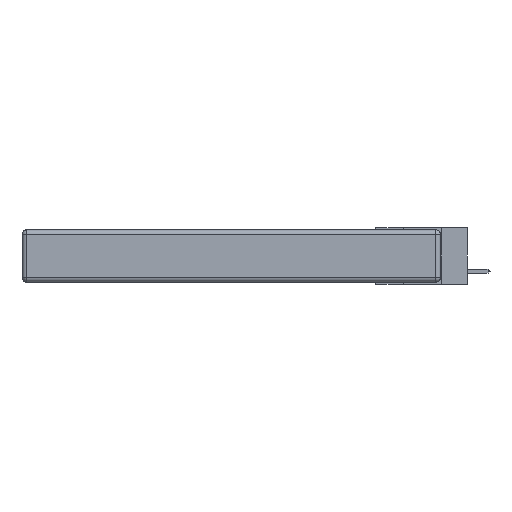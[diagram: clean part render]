
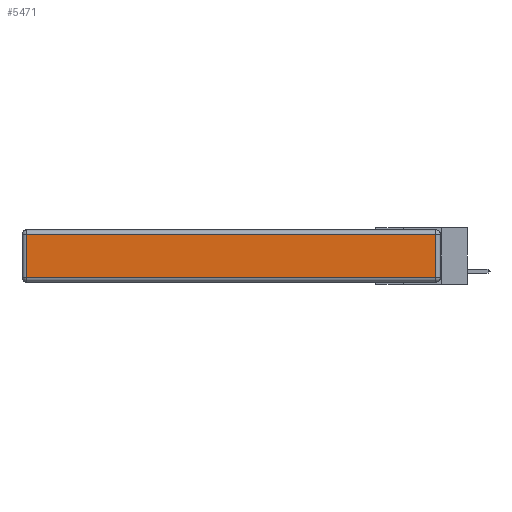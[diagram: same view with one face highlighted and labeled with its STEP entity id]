
A CAD part, left-side view. The second image highlights one B-rep face of the part: STEP entity #5471.
In plain terms, the highlighted planar face has unit normal (-1, 0, 0).
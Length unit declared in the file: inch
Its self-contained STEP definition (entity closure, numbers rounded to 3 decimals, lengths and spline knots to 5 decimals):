
#428 = CARTESIAN_POINT ( 'NONE',  ( 0., 0.03, -0.313 ) ) ;
#911 = EDGE_CURVE ( 'NONE', #13540, #8056, #10536, .T. ) ;
#1095 = VERTEX_POINT ( 'NONE', #428 ) ;
#1838 = ORIENTED_EDGE ( 'NONE', *, *, #20909, .T. ) ;
#2968 = CARTESIAN_POINT ( 'NONE',  ( 0., 2.72, -0.313 ) ) ;
#4421 = DIRECTION ( 'NONE',  ( 0., 1., 0. ) ) ;
#4935 = ORIENTED_EDGE ( 'NONE', *, *, #13201, .T. ) ;
#5303 = DIRECTION ( 'NONE',  ( -1., 0., 0. ) ) ;
#5471 = ADVANCED_FACE ( 'NONE', ( #12807 ), #6971, .T. ) ;
#5778 = AXIS2_PLACEMENT_3D ( 'NONE', #19087, #5303, #8729 ) ;
#5920 = VECTOR ( 'NONE', #4421, 39.37008 ) ;
#6203 = VECTOR ( 'NONE', #10778, 39.37008 ) ;
#6971 = PLANE ( 'NONE',  #5778 ) ;
#7053 = CARTESIAN_POINT ( 'NONE',  ( 0., 0.03, -0.343 ) ) ;
#7237 = CARTESIAN_POINT ( 'NONE',  ( 0., 0., -0.313 ) ) ;
#7710 = VECTOR ( 'NONE', #8641, 39.37008 ) ;
#8056 = VERTEX_POINT ( 'NONE', #19097 ) ;
#8262 = ORIENTED_EDGE ( 'NONE', *, *, #9685, .T. ) ;
#8641 = DIRECTION ( 'NONE',  ( 0., 0., 1. ) ) ;
#8729 = DIRECTION ( 'NONE',  ( 0., 0., 1. ) ) ;
#9056 = DIRECTION ( 'NONE',  ( 0., -1., 0. ) ) ;
#9260 = LINE ( 'NONE', #7237, #15230 ) ;
#9544 = CARTESIAN_POINT ( 'NONE',  ( 0., 2.75, -0.03 ) ) ;
#9685 = EDGE_CURVE ( 'NONE', #1095, #13540, #13701, .T. ) ;
#9986 = ORIENTED_EDGE ( 'NONE', *, *, #911, .T. ) ;
#10435 = CARTESIAN_POINT ( 'NONE',  ( 0., 0.03, -0.03 ) ) ;
#10536 = LINE ( 'NONE', #9544, #5920 ) ;
#10778 = DIRECTION ( 'NONE',  ( 0., 0., -1. ) ) ;
#10860 = CARTESIAN_POINT ( 'NONE',  ( 0., 2.72, -0.343 ) ) ;
#12807 = FACE_OUTER_BOUND ( 'NONE', #17669, .T. ) ;
#13201 = EDGE_CURVE ( 'NONE', #19943, #1095, #9260, .T. ) ;
#13540 = VERTEX_POINT ( 'NONE', #10435 ) ;
#13701 = LINE ( 'NONE', #7053, #7710 ) ;
#15230 = VECTOR ( 'NONE', #9056, 39.37008 ) ;
#15446 = LINE ( 'NONE', #10860, #6203 ) ;
#17669 = EDGE_LOOP ( 'NONE', ( #4935, #8262, #9986, #1838 ) ) ;
#19087 = CARTESIAN_POINT ( 'NONE',  ( 0., 0., -0.343 ) ) ;
#19097 = CARTESIAN_POINT ( 'NONE',  ( 0., 2.72, -0.03 ) ) ;
#19943 = VERTEX_POINT ( 'NONE', #2968 ) ;
#20909 = EDGE_CURVE ( 'NONE', #8056, #19943, #15446, .T. ) ;
